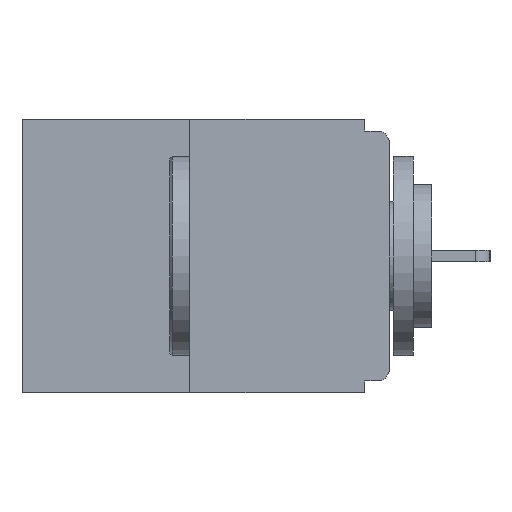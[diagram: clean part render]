
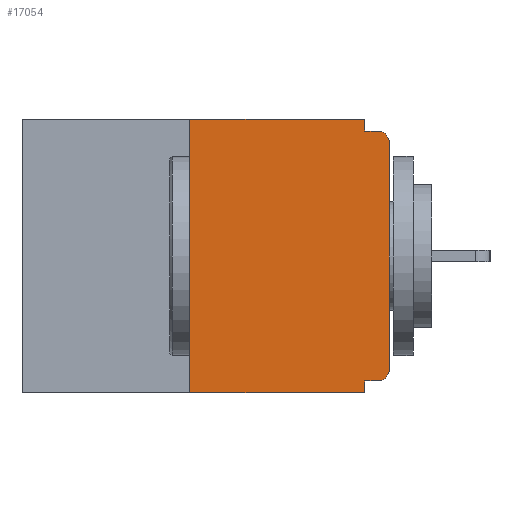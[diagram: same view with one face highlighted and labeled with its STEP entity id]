
A CAD part, left-side view. The second image highlights one B-rep face of the part: STEP entity #17054.
In plain terms, the highlighted planar face has unit normal (-1, 0, 0).
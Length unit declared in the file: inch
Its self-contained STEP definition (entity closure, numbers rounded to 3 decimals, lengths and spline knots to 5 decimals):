
#270 = VERTEX_POINT ( 'NONE', #24024 ) ;
#300 = DIRECTION ( 'NONE',  ( 0., 0., -1. ) ) ;
#819 = DIRECTION ( 'NONE',  ( 0., -1., 0. ) ) ;
#1081 = EDGE_CURVE ( 'NONE', #10633, #22162, #12253, .T. ) ;
#1222 = FACE_OUTER_BOUND ( 'NONE', #18931, .T. ) ;
#1287 = CARTESIAN_POINT ( 'NONE',  ( 0., 0.25, -0.343 ) ) ;
#1346 = DIRECTION ( 'NONE',  ( 0., -1., 0. ) ) ;
#1368 = VECTOR ( 'NONE', #1346, 39.37008 ) ;
#1481 = CARTESIAN_POINT ( 'NONE',  ( 0., 0.031, -0.343 ) ) ;
#1803 = VERTEX_POINT ( 'NONE', #13411 ) ;
#2641 = CARTESIAN_POINT ( 'NONE',  ( 0., 0.015, -0.313 ) ) ;
#3492 = VECTOR ( 'NONE', #300, 39.37008 ) ;
#3899 = LINE ( 'NONE', #11915, #1368 ) ;
#3985 = ORIENTED_EDGE ( 'NONE', *, *, #9615, .F. ) ;
#4006 = ORIENTED_EDGE ( 'NONE', *, *, #24659, .T. ) ;
#4568 = ORIENTED_EDGE ( 'NONE', *, *, #8083, .T. ) ;
#4739 = CARTESIAN_POINT ( 'NONE',  ( 0., 0.031, 0. ) ) ;
#4973 = LINE ( 'NONE', #15281, #15840 ) ;
#5075 = DIRECTION ( 'NONE',  ( 0., 1., 0. ) ) ;
#5123 = LINE ( 'NONE', #5400, #17810 ) ;
#5127 = VERTEX_POINT ( 'NONE', #17857 ) ;
#5145 = VERTEX_POINT ( 'NONE', #23781 ) ;
#5258 = CARTESIAN_POINT ( 'NONE',  ( 0., 0.46, 0. ) ) ;
#5400 = CARTESIAN_POINT ( 'NONE',  ( 0., 0.46, -0.343 ) ) ;
#5707 = CARTESIAN_POINT ( 'NONE',  ( 0., 0.46, 0. ) ) ;
#5721 = CARTESIAN_POINT ( 'NONE',  ( 0., 0., -0.03 ) ) ;
#6141 = CARTESIAN_POINT ( 'NONE',  ( 0., 0.015, -0.03 ) ) ;
#6371 = VERTEX_POINT ( 'NONE', #6917 ) ;
#6917 = CARTESIAN_POINT ( 'NONE',  ( 0., 0.031, -0.328 ) ) ;
#6943 = VECTOR ( 'NONE', #8232, 39.37008 ) ;
#7099 = DIRECTION ( 'NONE',  ( 0., 0., 1. ) ) ;
#7237 = EDGE_CURVE ( 'NONE', #18139, #5127, #5123, .T. ) ;
#7291 = ORIENTED_EDGE ( 'NONE', *, *, #19549, .T. ) ;
#7485 = AXIS2_PLACEMENT_3D ( 'NONE', #2641, #18885, #12972 ) ;
#8083 = EDGE_CURVE ( 'NONE', #18311, #270, #23880, .T. ) ;
#8102 = LINE ( 'NONE', #24519, #6943 ) ;
#8232 = DIRECTION ( 'NONE',  ( 0., 0., 1. ) ) ;
#8722 = VECTOR ( 'NONE', #9646, 39.37008 ) ;
#8900 = EDGE_CURVE ( 'NONE', #22162, #1803, #18559, .T. ) ;
#9267 = DIRECTION ( 'NONE',  ( 0., 0., -1. ) ) ;
#9615 = EDGE_CURVE ( 'NONE', #1803, #270, #3899, .T. ) ;
#9646 = DIRECTION ( 'NONE',  ( 0., 0., -1. ) ) ;
#10220 = AXIS2_PLACEMENT_3D ( 'NONE', #5258, #13694, #9267 ) ;
#10633 = VERTEX_POINT ( 'NONE', #26097 ) ;
#10679 = VECTOR ( 'NONE', #5075, 39.37008 ) ;
#11264 = PLANE ( 'NONE',  #10220 ) ;
#11638 = LINE ( 'NONE', #1481, #8722 ) ;
#11915 = CARTESIAN_POINT ( 'NONE',  ( 0., 0., -0.015 ) ) ;
#12244 = AXIS2_PLACEMENT_3D ( 'NONE', #6141, #14322, #20754 ) ;
#12253 = LINE ( 'NONE', #5707, #20079 ) ;
#12972 = DIRECTION ( 'NONE',  ( 0., 0., -1. ) ) ;
#13411 = CARTESIAN_POINT ( 'NONE',  ( 0., 0.031, -0.015 ) ) ;
#13507 = EDGE_CURVE ( 'NONE', #5145, #6371, #13637, .T. ) ;
#13637 = LINE ( 'NONE', #17664, #10679 ) ;
#13694 = DIRECTION ( 'NONE',  ( 1., 0., 0. ) ) ;
#14322 = DIRECTION ( 'NONE',  ( -1., 0., 0. ) ) ;
#15193 = CIRCLE ( 'NONE', #7485, 0.015 ) ;
#15227 = ORIENTED_EDGE ( 'NONE', *, *, #23945, .F. ) ;
#15269 = ORIENTED_EDGE ( 'NONE', *, *, #1081, .F. ) ;
#15281 = CARTESIAN_POINT ( 'NONE',  ( 0., 0.25, 0. ) ) ;
#15840 = VECTOR ( 'NONE', #7099, 39.37008 ) ;
#16237 = EDGE_CURVE ( 'NONE', #18139, #10633, #4973, .T. ) ;
#17054 = ADVANCED_FACE ( 'NONE', ( #1222 ), #11264, .F. ) ;
#17622 = ORIENTED_EDGE ( 'NONE', *, *, #13507, .F. ) ;
#17664 = CARTESIAN_POINT ( 'NONE',  ( 0., 0., -0.328 ) ) ;
#17810 = VECTOR ( 'NONE', #819, 39.37008 ) ;
#17857 = CARTESIAN_POINT ( 'NONE',  ( 0., 0.031, -0.343 ) ) ;
#18139 = VERTEX_POINT ( 'NONE', #1287 ) ;
#18311 = VERTEX_POINT ( 'NONE', #5721 ) ;
#18559 = LINE ( 'NONE', #4739, #3492 ) ;
#18885 = DIRECTION ( 'NONE',  ( -1., 0., 0. ) ) ;
#18931 = EDGE_LOOP ( 'NONE', ( #15269, #25973, #19093, #15227, #17622, #4006, #7291, #4568, #3985, #24542 ) ) ;
#19093 = ORIENTED_EDGE ( 'NONE', *, *, #7237, .T. ) ;
#19489 = CARTESIAN_POINT ( 'NONE',  ( 0., 0.031, 0. ) ) ;
#19549 = EDGE_CURVE ( 'NONE', #24850, #18311, #8102, .T. ) ;
#20079 = VECTOR ( 'NONE', #26241, 39.37008 ) ;
#20754 = DIRECTION ( 'NONE',  ( 0., 0., -1. ) ) ;
#22162 = VERTEX_POINT ( 'NONE', #19489 ) ;
#23781 = CARTESIAN_POINT ( 'NONE',  ( 0., 0.015, -0.328 ) ) ;
#23880 = CIRCLE ( 'NONE', #12244, 0.015 ) ;
#23896 = CARTESIAN_POINT ( 'NONE',  ( 0., 0., -0.313 ) ) ;
#23945 = EDGE_CURVE ( 'NONE', #6371, #5127, #11638, .T. ) ;
#24024 = CARTESIAN_POINT ( 'NONE',  ( 0., 0.015, -0.015 ) ) ;
#24519 = CARTESIAN_POINT ( 'NONE',  ( 0., 0., 0. ) ) ;
#24542 = ORIENTED_EDGE ( 'NONE', *, *, #8900, .F. ) ;
#24659 = EDGE_CURVE ( 'NONE', #5145, #24850, #15193, .T. ) ;
#24850 = VERTEX_POINT ( 'NONE', #23896 ) ;
#25973 = ORIENTED_EDGE ( 'NONE', *, *, #16237, .F. ) ;
#26097 = CARTESIAN_POINT ( 'NONE',  ( 0., 0.25, 0. ) ) ;
#26241 = DIRECTION ( 'NONE',  ( 0., -1., 0. ) ) ;
